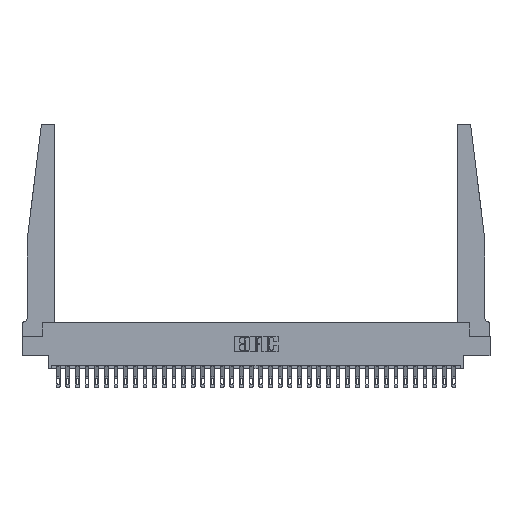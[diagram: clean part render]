
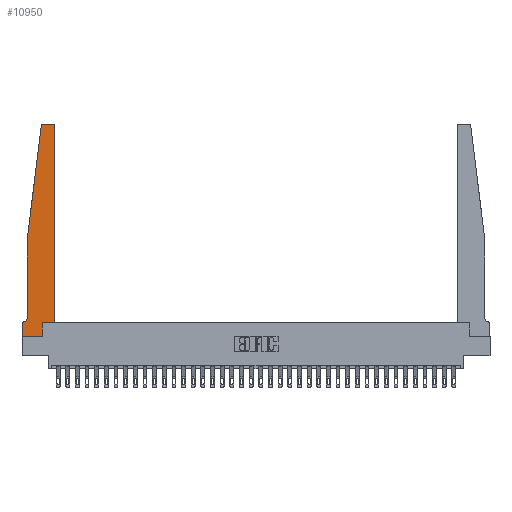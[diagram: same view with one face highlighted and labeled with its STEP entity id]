
A CAD part, top view. The second image highlights one B-rep face of the part: STEP entity #10950.
In plain terms, the highlighted planar face has unit normal (0, 0, 1).
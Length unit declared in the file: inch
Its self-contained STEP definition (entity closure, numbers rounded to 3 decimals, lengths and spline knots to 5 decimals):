
#241 = CARTESIAN_POINT ( 'NONE',  ( 0.065, 0.1875, 0.37 ) ) ;
#422 = CARTESIAN_POINT ( 'NONE',  ( 0., 0., 0.37 ) ) ;
#783 = VERTEX_POINT ( 'NONE', #32075 ) ;
#954 = ORIENTED_EDGE ( 'NONE', *, *, #1033, .T. ) ;
#1033 = EDGE_CURVE ( 'NONE', #783, #6229, #19077, .T. ) ;
#1051 = LINE ( 'NONE', #28574, #26348 ) ;
#1664 = CARTESIAN_POINT ( 'NONE',  ( 0.2605, 0.18, 0.37 ) ) ;
#1703 = VECTOR ( 'NONE', #31144, 39.37008 ) ;
#1921 = AXIS2_PLACEMENT_3D ( 'NONE', #32067, #22059, #6937 ) ;
#2604 = VERTEX_POINT ( 'NONE', #5853 ) ;
#3014 = CARTESIAN_POINT ( 'NONE',  ( 0.425, 2.72, 0.37 ) ) ;
#3411 = DIRECTION ( 'NONE',  ( 0., -1., 0. ) ) ;
#3991 = ORIENTED_EDGE ( 'NONE', *, *, #11855, .T. ) ;
#4133 = DIRECTION ( 'NONE',  ( 0., 0., 1. ) ) ;
#4168 = VERTEX_POINT ( 'NONE', #6844 ) ;
#4419 = PLANE ( 'NONE',  #1921 ) ;
#4594 = VECTOR ( 'NONE', #12402, 39.37008 ) ;
#5048 = LINE ( 'NONE', #241, #23605 ) ;
#5262 = ORIENTED_EDGE ( 'NONE', *, *, #20590, .T. ) ;
#5295 = VECTOR ( 'NONE', #11683, 39.37008 ) ;
#5853 = CARTESIAN_POINT ( 'NONE',  ( 0.065, 0.2375, 0.37 ) ) ;
#6229 = VERTEX_POINT ( 'NONE', #29538 ) ;
#6844 = CARTESIAN_POINT ( 'NONE',  ( 0.395, 2.75, 0.37 ) ) ;
#6937 = DIRECTION ( 'NONE',  ( 1., 0., 0. ) ) ;
#7064 = CIRCLE ( 'NONE', #29463, 0.03 ) ;
#7462 = ORIENTED_EDGE ( 'NONE', *, *, #15701, .T. ) ;
#7719 = ORIENTED_EDGE ( 'NONE', *, *, #8840, .T. ) ;
#7895 = DIRECTION ( 'NONE',  ( 0., 0., -1. ) ) ;
#8419 = LINE ( 'NONE', #16106, #1703 ) ;
#8671 = CARTESIAN_POINT ( 'NONE',  ( 0., 0.1875, 0.37 ) ) ;
#8840 = EDGE_CURVE ( 'NONE', #10411, #25186, #23479, .T. ) ;
#9224 = DIRECTION ( 'NONE',  ( -0.122, -0.992, 0. ) ) ;
#10411 = VERTEX_POINT ( 'NONE', #27391 ) ;
#10431 = DIRECTION ( 'NONE',  ( -1., 0., 0. ) ) ;
#10655 = EDGE_LOOP ( 'NONE', ( #5262, #7719, #29771, #26758, #3991, #7462, #24989, #954, #11351, #29460, #26782, #30432 ) ) ;
#10950 = ADVANCED_FACE ( 'NONE', ( #20993 ), #4419, .T. ) ;
#11351 = ORIENTED_EDGE ( 'NONE', *, *, #16079, .T. ) ;
#11387 = CARTESIAN_POINT ( 'NONE',  ( 0.425, 0.18, 0.37 ) ) ;
#11683 = DIRECTION ( 'NONE',  ( -1., 0., 0. ) ) ;
#11855 = EDGE_CURVE ( 'NONE', #2604, #23021, #27648, .T. ) ;
#12046 = LINE ( 'NONE', #26770, #5295 ) ;
#12402 = DIRECTION ( 'NONE',  ( 0., -1., 0. ) ) ;
#12532 = AXIS2_PLACEMENT_3D ( 'NONE', #22998, #7895, #25552 ) ;
#13324 = DIRECTION ( 'NONE',  ( 0., 0., 1. ) ) ;
#13666 = LINE ( 'NONE', #28454, #14461 ) ;
#14461 = VECTOR ( 'NONE', #30941, 39.37008 ) ;
#14867 = EDGE_CURVE ( 'NONE', #26810, #4168, #7064, .T. ) ;
#15287 = CARTESIAN_POINT ( 'NONE',  ( 0.065, 1.25, 0.37 ) ) ;
#15701 = EDGE_CURVE ( 'NONE', #23021, #23099, #5048, .T. ) ;
#16079 = EDGE_CURVE ( 'NONE', #6229, #16889, #26746, .T. ) ;
#16106 = CARTESIAN_POINT ( 'NONE',  ( 0.425, 0.18, 0.37 ) ) ;
#16806 = DIRECTION ( 'NONE',  ( 0., 1., 0. ) ) ;
#16889 = VERTEX_POINT ( 'NONE', #27870 ) ;
#17538 = VERTEX_POINT ( 'NONE', #15287 ) ;
#17766 = LINE ( 'NONE', #24322, #31150 ) ;
#18119 = DIRECTION ( 'NONE',  ( 1., 0., 0. ) ) ;
#19077 = LINE ( 'NONE', #422, #19883 ) ;
#19241 = CARTESIAN_POINT ( 'NONE',  ( 0.27653, 2.72, 0.37 ) ) ;
#19883 = VECTOR ( 'NONE', #18119, 39.37008 ) ;
#20137 = VERTEX_POINT ( 'NONE', #11387 ) ;
#20590 = EDGE_CURVE ( 'NONE', #4168, #10411, #12046, .T. ) ;
#20993 = FACE_OUTER_BOUND ( 'NONE', #10655, .T. ) ;
#21768 = DIRECTION ( 'NONE',  ( 1., 0., 0. ) ) ;
#22059 = DIRECTION ( 'NONE',  ( 0., 0., 1. ) ) ;
#22998 = CARTESIAN_POINT ( 'NONE',  ( 0.015, 0.2375, 0.37 ) ) ;
#23021 = VERTEX_POINT ( 'NONE', #31042 ) ;
#23099 = VERTEX_POINT ( 'NONE', #8671 ) ;
#23228 = EDGE_CURVE ( 'NONE', #25186, #17538, #17766, .T. ) ;
#23479 = CIRCLE ( 'NONE', #31654, 0.03 ) ;
#23605 = VECTOR ( 'NONE', #10431, 39.37008 ) ;
#24322 = CARTESIAN_POINT ( 'NONE',  ( 0.065, 1.25, 0.37 ) ) ;
#24856 = EDGE_CURVE ( 'NONE', #23099, #783, #1051, .T. ) ;
#24989 = ORIENTED_EDGE ( 'NONE', *, *, #24856, .T. ) ;
#25186 = VERTEX_POINT ( 'NONE', #27218 ) ;
#25487 = EDGE_CURVE ( 'NONE', #20137, #26810, #8419, .T. ) ;
#25552 = DIRECTION ( 'NONE',  ( -1., 0., 0. ) ) ;
#26329 = LINE ( 'NONE', #29923, #4594 ) ;
#26348 = VECTOR ( 'NONE', #3411, 39.37008 ) ;
#26746 = LINE ( 'NONE', #1664, #28339 ) ;
#26758 = ORIENTED_EDGE ( 'NONE', *, *, #30114, .T. ) ;
#26770 = CARTESIAN_POINT ( 'NONE',  ( 0.25, 2.75, 0.37 ) ) ;
#26782 = ORIENTED_EDGE ( 'NONE', *, *, #25487, .T. ) ;
#26810 = VERTEX_POINT ( 'NONE', #3014 ) ;
#27218 = CARTESIAN_POINT ( 'NONE',  ( 0.24675, 2.72367, 0.37 ) ) ;
#27391 = CARTESIAN_POINT ( 'NONE',  ( 0.27653, 2.75, 0.37 ) ) ;
#27648 = CIRCLE ( 'NONE', #12532, 0.05 ) ;
#27870 = CARTESIAN_POINT ( 'NONE',  ( 0.2605, 0.18, 0.37 ) ) ;
#28339 = VECTOR ( 'NONE', #16806, 39.37008 ) ;
#28404 = CARTESIAN_POINT ( 'NONE',  ( 0.395, 2.72, 0.37 ) ) ;
#28454 = CARTESIAN_POINT ( 'NONE',  ( 0.425, 0.18, 0.37 ) ) ;
#28574 = CARTESIAN_POINT ( 'NONE',  ( 0., 0., 0.37 ) ) ;
#29460 = ORIENTED_EDGE ( 'NONE', *, *, #30947, .T. ) ;
#29463 = AXIS2_PLACEMENT_3D ( 'NONE', #28404, #13324, #30891 ) ;
#29538 = CARTESIAN_POINT ( 'NONE',  ( 0.2605, 0., 0.37 ) ) ;
#29771 = ORIENTED_EDGE ( 'NONE', *, *, #23228, .T. ) ;
#29923 = CARTESIAN_POINT ( 'NONE',  ( 0.065, 1.25, 0.37 ) ) ;
#30114 = EDGE_CURVE ( 'NONE', #17538, #2604, #26329, .T. ) ;
#30432 = ORIENTED_EDGE ( 'NONE', *, *, #14867, .T. ) ;
#30891 = DIRECTION ( 'NONE',  ( 1., 0., 0. ) ) ;
#30941 = DIRECTION ( 'NONE',  ( 1., 0., 0. ) ) ;
#30947 = EDGE_CURVE ( 'NONE', #16889, #20137, #13666, .T. ) ;
#31042 = CARTESIAN_POINT ( 'NONE',  ( 0.015, 0.1875, 0.37 ) ) ;
#31144 = DIRECTION ( 'NONE',  ( 0., 1., 0. ) ) ;
#31150 = VECTOR ( 'NONE', #9224, 39.37008 ) ;
#31654 = AXIS2_PLACEMENT_3D ( 'NONE', #19241, #4133, #21768 ) ;
#32067 = CARTESIAN_POINT ( 'NONE',  ( 0., 0.1875, 0.37 ) ) ;
#32075 = CARTESIAN_POINT ( 'NONE',  ( 0., 0., 0.37 ) ) ;
